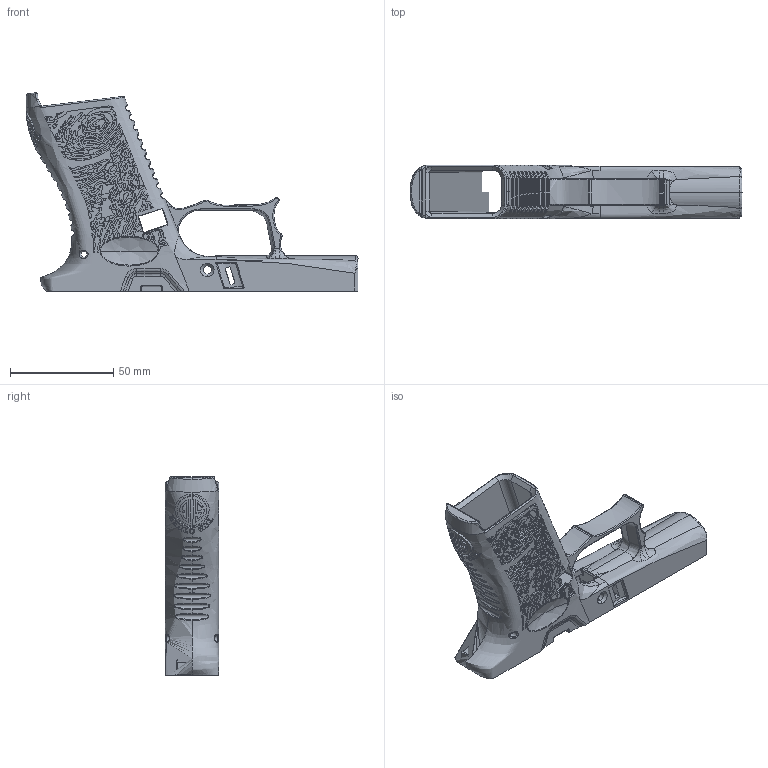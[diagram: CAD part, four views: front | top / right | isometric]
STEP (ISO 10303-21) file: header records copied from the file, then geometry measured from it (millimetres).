
FILE_DESCRIPTION (( 'STEP AP203' ), '1' );
FILE_NAME ('43X D.A.N. FDM.STEP', '2020-12-17T00:58:41', ( '' ), ( '' ), 'SwSTEP 2.0', 'SolidWorks 2016', '' );
FILE_SCHEMA (( 'CONFIG_CONTROL_DESIGN' ));
Products named in the file (1): 43X D.A.N. FDM
Bounding box: 160.56 x 25.9 x 95.92 mm (x, y, z)
Volume: 61922.9 mm3; surface area: 41643.4 mm2
Topology: 1 solids, 1 shells, 2571 faces, 6798 edges, 4379 vertices
Faces by surface type: bspline 1565, plane 590, cylinder 376, torus 26, cone 12, sphere 2
Entity records: 518341 total; most frequent: CARTESIAN_POINT 467625, ORIENTED_EDGE 13524, EDGE_CURVE 6762, DIRECTION 5225, VERTEX_POINT 4379, B_SPLINE_CURVE_WITH_KNOTS 3962, EDGE_LOOP 2779, ADVANCED_FACE 2571
